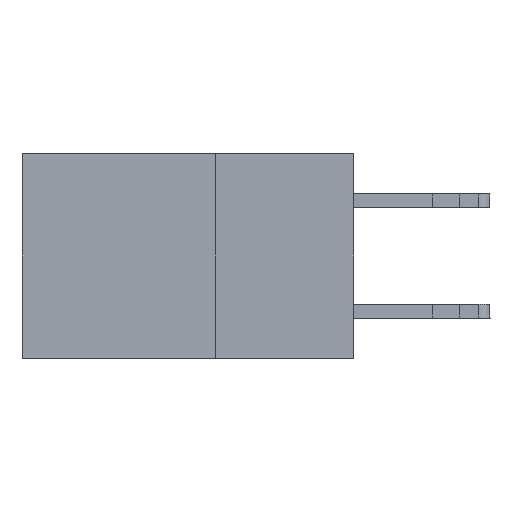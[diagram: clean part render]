
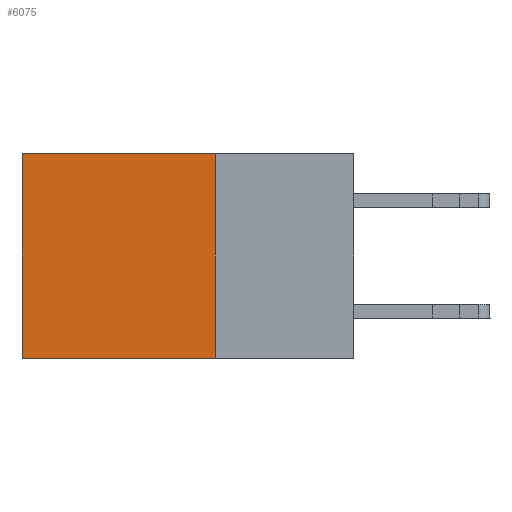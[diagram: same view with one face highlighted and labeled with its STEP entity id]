
A CAD part, left-side view. The second image highlights one B-rep face of the part: STEP entity #6075.
In plain terms, the highlighted planar face has unit normal (-1, 0, 0).
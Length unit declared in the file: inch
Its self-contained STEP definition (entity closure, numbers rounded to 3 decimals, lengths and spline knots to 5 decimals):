
#39 = DIRECTION ( 'NONE',  ( 0., 1., 0. ) ) ;
#802 = CARTESIAN_POINT ( 'NONE',  ( 0.2875, 0.25, -0.37 ) ) ;
#1202 = CARTESIAN_POINT ( 'NONE',  ( 0.2875, 0.6, -0.37 ) ) ;
#1393 = VECTOR ( 'NONE', #5545, 39.37008 ) ;
#1430 = ORIENTED_EDGE ( 'NONE', *, *, #15665, .F. ) ;
#3487 = PLANE ( 'NONE',  #4569 ) ;
#4569 = AXIS2_PLACEMENT_3D ( 'NONE', #5505, #18388, #20869 ) ;
#5505 = CARTESIAN_POINT ( 'NONE',  ( 0.2875, 0.25, 0. ) ) ;
#5545 = DIRECTION ( 'NONE',  ( 0., 0., -1. ) ) ;
#6075 = ADVANCED_FACE ( 'NONE', ( #12572 ), #3487, .F. ) ;
#6188 = VECTOR ( 'NONE', #17915, 39.37008 ) ;
#6450 = LINE ( 'NONE', #12108, #7782 ) ;
#7084 = VERTEX_POINT ( 'NONE', #15877 ) ;
#7603 = LINE ( 'NONE', #19074, #22092 ) ;
#7782 = VECTOR ( 'NONE', #21671, 39.37008 ) ;
#7878 = ORIENTED_EDGE ( 'NONE', *, *, #12828, .T. ) ;
#10027 = CARTESIAN_POINT ( 'NONE',  ( 0.2875, 0.6, 0. ) ) ;
#10955 = CARTESIAN_POINT ( 'NONE',  ( 0.2875, 0.25, 0. ) ) ;
#12108 = CARTESIAN_POINT ( 'NONE',  ( 0.2875, 0.6, 0. ) ) ;
#12114 = LINE ( 'NONE', #19804, #6188 ) ;
#12572 = FACE_OUTER_BOUND ( 'NONE', #24387, .T. ) ;
#12828 = EDGE_CURVE ( 'NONE', #20877, #21968, #6450, .T. ) ;
#15114 = EDGE_CURVE ( 'NONE', #19570, #21968, #12114, .T. ) ;
#15665 = EDGE_CURVE ( 'NONE', #7084, #19570, #24676, .T. ) ;
#15762 = ORIENTED_EDGE ( 'NONE', *, *, #22563, .T. ) ;
#15877 = CARTESIAN_POINT ( 'NONE',  ( 0.2875, 0.25, 0. ) ) ;
#17915 = DIRECTION ( 'NONE',  ( 0., 1., 0. ) ) ;
#18388 = DIRECTION ( 'NONE',  ( 1., 0., 0. ) ) ;
#19074 = CARTESIAN_POINT ( 'NONE',  ( 0.2875, 0.25, 0. ) ) ;
#19570 = VERTEX_POINT ( 'NONE', #802 ) ;
#19804 = CARTESIAN_POINT ( 'NONE',  ( 0.2875, 0.25, -0.37 ) ) ;
#20869 = DIRECTION ( 'NONE',  ( 0., 0., -1. ) ) ;
#20877 = VERTEX_POINT ( 'NONE', #10027 ) ;
#21671 = DIRECTION ( 'NONE',  ( 0., 0., -1. ) ) ;
#21879 = ORIENTED_EDGE ( 'NONE', *, *, #15114, .F. ) ;
#21968 = VERTEX_POINT ( 'NONE', #1202 ) ;
#22092 = VECTOR ( 'NONE', #39, 39.37008 ) ;
#22563 = EDGE_CURVE ( 'NONE', #7084, #20877, #7603, .T. ) ;
#24387 = EDGE_LOOP ( 'NONE', ( #7878, #21879, #1430, #15762 ) ) ;
#24676 = LINE ( 'NONE', #10955, #1393 ) ;
